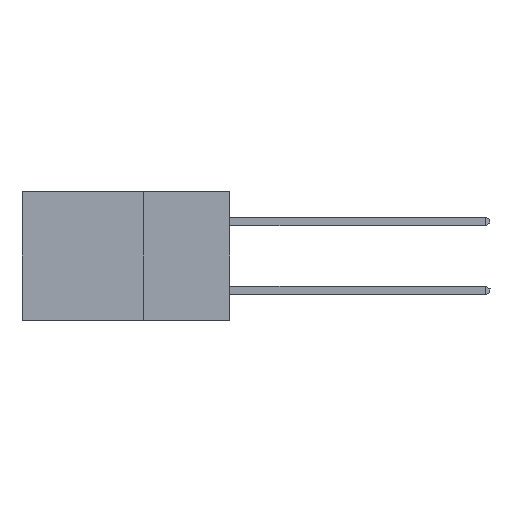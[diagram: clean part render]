
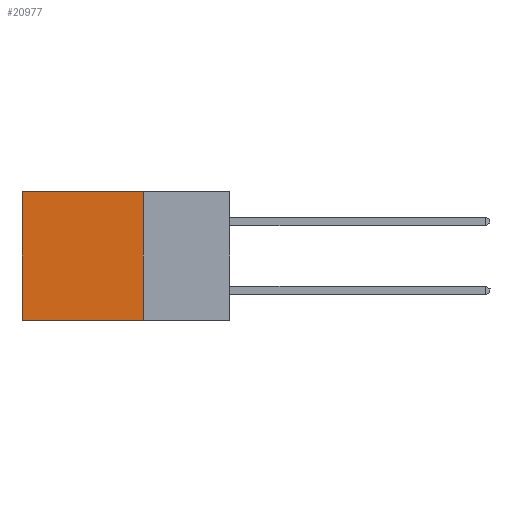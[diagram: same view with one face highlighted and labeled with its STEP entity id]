
A CAD part, left-side view. The second image highlights one B-rep face of the part: STEP entity #20977.
In plain terms, the highlighted planar face has unit normal (-1, 0, 0).
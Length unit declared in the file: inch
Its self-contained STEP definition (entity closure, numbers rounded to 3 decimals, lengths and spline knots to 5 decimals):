
#388 = VERTEX_POINT ( 'NONE', #3909 ) ;
#637 = CARTESIAN_POINT ( 'NONE',  ( 0.298, 0.6, -0.37 ) ) ;
#967 = LINE ( 'NONE', #1016, #16819 ) ;
#1016 = CARTESIAN_POINT ( 'NONE',  ( 0.298, 0.6, 0. ) ) ;
#2104 = VERTEX_POINT ( 'NONE', #19914 ) ;
#2777 = ORIENTED_EDGE ( 'NONE', *, *, #24199, .T. ) ;
#3909 = CARTESIAN_POINT ( 'NONE',  ( 0.298, 0.6, 0. ) ) ;
#5802 = VECTOR ( 'NONE', #12367, 39.37008 ) ;
#8365 = CARTESIAN_POINT ( 'NONE',  ( 0.298, 0.25, 0. ) ) ;
#9116 = VERTEX_POINT ( 'NONE', #637 ) ;
#9290 = AXIS2_PLACEMENT_3D ( 'NONE', #11151, #20792, #17156 ) ;
#9438 = VECTOR ( 'NONE', #23862, 39.37008 ) ;
#10226 = ORIENTED_EDGE ( 'NONE', *, *, #15363, .F. ) ;
#10492 = ORIENTED_EDGE ( 'NONE', *, *, #14202, .T. ) ;
#11151 = CARTESIAN_POINT ( 'NONE',  ( 0.298, 0.25, 0. ) ) ;
#11180 = VECTOR ( 'NONE', #21703, 39.37008 ) ;
#12367 = DIRECTION ( 'NONE',  ( 0., 1., 0. ) ) ;
#12386 = EDGE_LOOP ( 'NONE', ( #10492, #13684, #10226, #2777 ) ) ;
#13684 = ORIENTED_EDGE ( 'NONE', *, *, #15331, .F. ) ;
#14137 = FACE_OUTER_BOUND ( 'NONE', #12386, .T. ) ;
#14202 = EDGE_CURVE ( 'NONE', #388, #9116, #967, .T. ) ;
#15331 = EDGE_CURVE ( 'NONE', #25098, #9116, #22278, .T. ) ;
#15363 = EDGE_CURVE ( 'NONE', #2104, #25098, #21958, .T. ) ;
#15829 = CARTESIAN_POINT ( 'NONE',  ( 0.298, 0.25, 0. ) ) ;
#16819 = VECTOR ( 'NONE', #18164, 39.37008 ) ;
#17156 = DIRECTION ( 'NONE',  ( 0., 0., -1. ) ) ;
#18164 = DIRECTION ( 'NONE',  ( 0., 0., -1. ) ) ;
#19914 = CARTESIAN_POINT ( 'NONE',  ( 0.298, 0.25, 0. ) ) ;
#20792 = DIRECTION ( 'NONE',  ( 1., 0., 0. ) ) ;
#20977 = ADVANCED_FACE ( 'NONE', ( #14137 ), #24611, .F. ) ;
#21703 = DIRECTION ( 'NONE',  ( 0., 1., 0. ) ) ;
#21958 = LINE ( 'NONE', #8365, #9438 ) ;
#22090 = CARTESIAN_POINT ( 'NONE',  ( 0.298, 0.25, -0.37 ) ) ;
#22278 = LINE ( 'NONE', #24036, #5802 ) ;
#22456 = LINE ( 'NONE', #15829, #11180 ) ;
#23862 = DIRECTION ( 'NONE',  ( 0., 0., -1. ) ) ;
#24036 = CARTESIAN_POINT ( 'NONE',  ( 0.298, 0.25, -0.37 ) ) ;
#24199 = EDGE_CURVE ( 'NONE', #2104, #388, #22456, .T. ) ;
#24611 = PLANE ( 'NONE',  #9290 ) ;
#25098 = VERTEX_POINT ( 'NONE', #22090 ) ;
